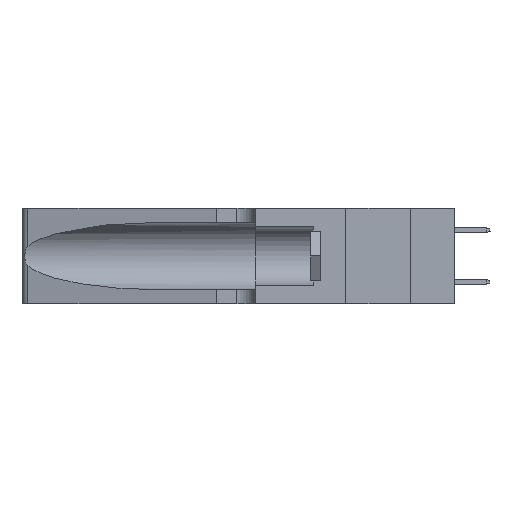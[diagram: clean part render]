
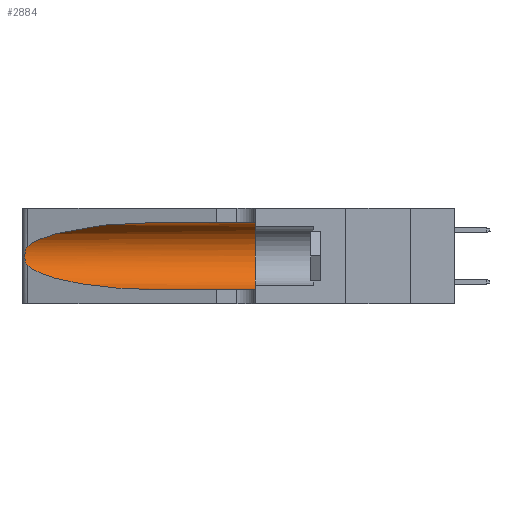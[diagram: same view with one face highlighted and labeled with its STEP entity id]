
A CAD part, left-side view. The second image highlights one B-rep face of the part: STEP entity #2884.
In plain terms, the highlighted cylindrical face has radius 3.308 mm (diameter 6.617 mm), a partial arc.
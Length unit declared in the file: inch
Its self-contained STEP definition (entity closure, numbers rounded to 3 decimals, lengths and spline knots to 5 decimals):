
#2068 = EDGE_CURVE ( 'NONE', #32809, #44559, #45009, .T. ) ;
#2390 = CYLINDRICAL_SURFACE ( 'NONE', #10717, 0.13025 ) ;
#2582 = EDGE_CURVE ( 'NONE', #3914, #6385, #9518, .T. ) ;
#2884 = ADVANCED_FACE ( 'NONE', ( #37866 ), #2390, .F. ) ;
#3914 = VERTEX_POINT ( 'NONE', #3996 ) ;
#3996 = CARTESIAN_POINT ( 'NONE',  ( 0.1305, 0.72297, 0.05475 ) ) ;
#6055 = CARTESIAN_POINT ( 'NONE',  ( 0.25487, 1.22718, 0.22369 ) ) ;
#6382 = CARTESIAN_POINT ( 'NONE',  ( 0.1305, 0.72297, 0.05475 ) ) ;
#6385 = VERTEX_POINT ( 'NONE', #23355 ) ;
#6548 = CARTESIAN_POINT ( 'NONE',  ( 0.25639, 1.23184, 0.21858 ) ) ;
#8221 = DIRECTION ( 'NONE',  ( 0., 1., 0. ) ) ;
#8255 = VECTOR ( 'NONE', #38414, 39.37008 ) ;
#8336 = CARTESIAN_POINT ( 'NONE',  ( 0.25856, 1.23593, 0.16098 ) ) ;
#8960 = B_SPLINE_CURVE_WITH_KNOTS ( 'NONE', 3,
 ( #27722, #27938, #6548, #13840, #17609, #28383, #26205, #29251, #15170, #8336, #18462, #33478, #11181, #25971 ),
 .UNSPECIFIED., .F., .F.,
 ( 4, 2, 2, 2, 2, 2, 4 ),
 ( 0., 0.00027, 0.00053, 0.00107, 0.0016, 0.00187, 0.00214 ),
 .UNSPECIFIED. ) ;
#9518 = LINE ( 'NONE', #45454, #18188 ) ;
#9926 = CARTESIAN_POINT ( 'NONE',  ( 0.25487, 1.22718, 0.14631 ) ) ;
#10518 = CARTESIAN_POINT ( 'NONE',  ( 0.18966, 0.96281, 0.31525 ) ) ;
#10717 = AXIS2_PLACEMENT_3D ( 'NONE', #35037, #34101, #27065 ) ;
#10869 = CIRCLE ( 'NONE', #33353, 0.13025 ) ;
#11181 = CARTESIAN_POINT ( 'NONE',  ( 0.25555, 1.22993, 0.14849 ) ) ;
#13840 = CARTESIAN_POINT ( 'NONE',  ( 0.25787, 1.23484, 0.2124 ) ) ;
#14035 = CARTESIAN_POINT ( 'NONE',  ( 0.1305, 0.72297, 0.31525 ) ) ;
#15170 = CARTESIAN_POINT ( 'NONE',  ( 0.26017, 1.23833, 0.17102 ) ) ;
#15261 = VERTEX_POINT ( 'NONE', #38417 ) ;
#17124 = EDGE_CURVE ( 'NONE', #32809, #19873, #45257, .T. ) ;
#17609 = CARTESIAN_POINT ( 'NONE',  ( 0.25854, 1.2359, 0.20912 ) ) ;
#18188 = VECTOR ( 'NONE', #43324, 39.37008 ) ;
#18462 = CARTESIAN_POINT ( 'NONE',  ( 0.25789, 1.23486, 0.15765 ) ) ;
#18824 = ORIENTED_EDGE ( 'NONE', *, *, #39145, .T. ) ;
#19873 = VERTEX_POINT ( 'NONE', #34984 ) ;
#22545 = DIRECTION ( 'NONE',  ( 0., 0., 1. ) ) ;
#23278 = CARTESIAN_POINT ( 'NONE',  ( 0.1305, 0.72297, 0.31525 ) ) ;
#23355 = CARTESIAN_POINT ( 'NONE',  ( 0.1305, 0.35, 0.05475 ) ) ;
#23923 = CARTESIAN_POINT ( 'NONE',  ( 0.2373, 1.15595, 0.28018 ) ) ;
#24090 = CARTESIAN_POINT ( 'NONE',  ( 0.1305, 1.61858, 0.31525 ) ) ;
#24257 = CARTESIAN_POINT ( 'NONE',  ( 0.2373, 1.15595, 0.08982 ) ) ;
#24278 = EDGE_CURVE ( 'NONE', #44559, #15261, #8960, .T. ) ;
#25971 = CARTESIAN_POINT ( 'NONE',  ( 0.25487, 1.22718, 0.14631 ) ) ;
#26205 = CARTESIAN_POINT ( 'NONE',  ( 0.26075, 1.23896, 0.19203 ) ) ;
#27065 = DIRECTION ( 'NONE',  ( 0., 0., -1. ) ) ;
#27722 = CARTESIAN_POINT ( 'NONE',  ( 0.25487, 1.22718, 0.22369 ) ) ;
#27938 = CARTESIAN_POINT ( 'NONE',  ( 0.25555, 1.22994, 0.2215 ) ) ;
#28383 = CARTESIAN_POINT ( 'NONE',  ( 0.26018, 1.23835, 0.19895 ) ) ;
#28557 = EDGE_LOOP ( 'NONE', ( #35369, #40772, #18824, #42640, #43420, #45966 ) ) ;
#29251 = CARTESIAN_POINT ( 'NONE',  ( 0.26075, 1.23896, 0.178 ) ) ;
#32809 = VERTEX_POINT ( 'NONE', #23278 ) ;
#33353 = AXIS2_PLACEMENT_3D ( 'NONE', #40421, #8221, #22545 ) ;
#33478 = CARTESIAN_POINT ( 'NONE',  ( 0.25639, 1.23186, 0.15144 ) ) ;
#33593 =( BOUNDED_CURVE ( )  B_SPLINE_CURVE ( 3, ( #9926, #24257, #38569, #6382 ),
 .UNSPECIFIED., .F., .T. ) 
 B_SPLINE_CURVE_WITH_KNOTS ( ( 4, 4 ),
 ( 3.44316, 4.71239 ),
 .UNSPECIFIED. ) 
 CURVE ( )  GEOMETRIC_REPRESENTATION_ITEM ( )  RATIONAL_B_SPLINE_CURVE ( ( 1., 0.87, 0.87, 1. ) ) 
 REPRESENTATION_ITEM ( '' )  );
#34101 = DIRECTION ( 'NONE',  ( 0., -1., 0. ) ) ;
#34984 = CARTESIAN_POINT ( 'NONE',  ( 0.1305, 0.35, 0.31525 ) ) ;
#35037 = CARTESIAN_POINT ( 'NONE',  ( 0.1305, 1.61858, 0.185 ) ) ;
#35369 = ORIENTED_EDGE ( 'NONE', *, *, #2068, .T. ) ;
#37866 = FACE_OUTER_BOUND ( 'NONE', #28557, .T. ) ;
#38414 = DIRECTION ( 'NONE',  ( 0., -1., 0. ) ) ;
#38417 = CARTESIAN_POINT ( 'NONE',  ( 0.25487, 1.22718, 0.14631 ) ) ;
#38569 = CARTESIAN_POINT ( 'NONE',  ( 0.18966, 0.96281, 0.05475 ) ) ;
#39145 = EDGE_CURVE ( 'NONE', #15261, #3914, #33593, .T. ) ;
#40421 = CARTESIAN_POINT ( 'NONE',  ( 0.1305, 0.35, 0.185 ) ) ;
#40772 = ORIENTED_EDGE ( 'NONE', *, *, #24278, .T. ) ;
#41137 = CARTESIAN_POINT ( 'NONE',  ( 0.25487, 1.22718, 0.22369 ) ) ;
#42640 = ORIENTED_EDGE ( 'NONE', *, *, #2582, .T. ) ;
#43006 = EDGE_CURVE ( 'NONE', #19873, #6385, #10869, .T. ) ;
#43324 = DIRECTION ( 'NONE',  ( 0., -1., 0. ) ) ;
#43420 = ORIENTED_EDGE ( 'NONE', *, *, #43006, .F. ) ;
#44559 = VERTEX_POINT ( 'NONE', #41137 ) ;
#45009 =( BOUNDED_CURVE ( )  B_SPLINE_CURVE ( 3, ( #14035, #10518, #23923, #6055 ),
 .UNSPECIFIED., .F., .T. ) 
 B_SPLINE_CURVE_WITH_KNOTS ( ( 4, 4 ),
 ( 1.5708, 2.84003 ),
 .UNSPECIFIED. ) 
 CURVE ( )  GEOMETRIC_REPRESENTATION_ITEM ( )  RATIONAL_B_SPLINE_CURVE ( ( 1., 0.87, 0.87, 1. ) ) 
 REPRESENTATION_ITEM ( '' )  );
#45257 = LINE ( 'NONE', #24090, #8255 ) ;
#45454 = CARTESIAN_POINT ( 'NONE',  ( 0.1305, 1.61858, 0.05475 ) ) ;
#45966 = ORIENTED_EDGE ( 'NONE', *, *, #17124, .F. ) ;
